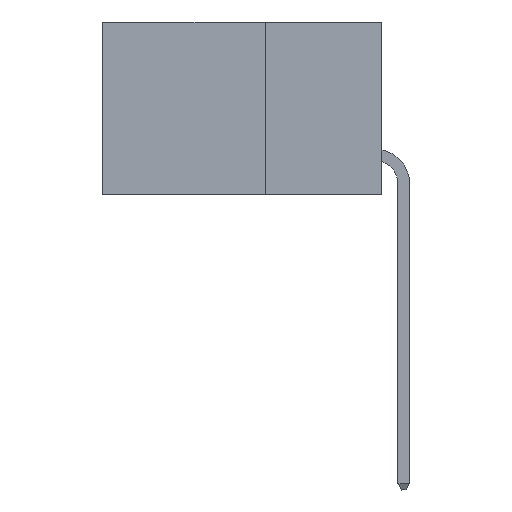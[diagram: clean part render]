
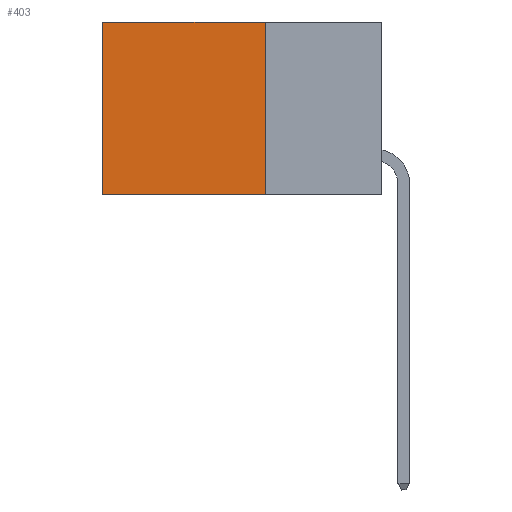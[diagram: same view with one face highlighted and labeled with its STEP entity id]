
A CAD part, left-side view. The second image highlights one B-rep face of the part: STEP entity #403.
In plain terms, the highlighted planar face has unit normal (-1, 0, 0).
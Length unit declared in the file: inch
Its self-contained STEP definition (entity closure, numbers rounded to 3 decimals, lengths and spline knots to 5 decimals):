
#159 = VERTEX_POINT ( 'NONE', #13754 ) ;
#403 = ADVANCED_FACE ( 'NONE', ( #7611 ), #3947, .F. ) ;
#595 = DIRECTION ( 'NONE',  ( 0., 0., -1. ) ) ;
#725 = DIRECTION ( 'NONE',  ( 1., 0., 0. ) ) ;
#1408 = VERTEX_POINT ( 'NONE', #18334 ) ;
#2193 = DIRECTION ( 'NONE',  ( 0., 0., -1. ) ) ;
#3204 = AXIS2_PLACEMENT_3D ( 'NONE', #6863, #725, #595 ) ;
#3571 = VECTOR ( 'NONE', #10130, 39.37008 ) ;
#3947 = PLANE ( 'NONE',  #3204 ) ;
#4691 = ORIENTED_EDGE ( 'NONE', *, *, #5246, .T. ) ;
#4752 = ORIENTED_EDGE ( 'NONE', *, *, #5936, .F. ) ;
#5246 = EDGE_CURVE ( 'NONE', #159, #1408, #19019, .T. ) ;
#5570 = LINE ( 'NONE', #14138, #19491 ) ;
#5896 = EDGE_LOOP ( 'NONE', ( #15686, #10786, #4752, #4691 ) ) ;
#5936 = EDGE_CURVE ( 'NONE', #159, #8295, #5570, .T. ) ;
#6798 = EDGE_CURVE ( 'NONE', #8295, #16236, #13762, .T. ) ;
#6863 = CARTESIAN_POINT ( 'NONE',  ( 0.2875, 0.25, 0. ) ) ;
#6903 = VECTOR ( 'NONE', #2193, 39.37008 ) ;
#7611 = FACE_OUTER_BOUND ( 'NONE', #5896, .T. ) ;
#8295 = VERTEX_POINT ( 'NONE', #10831 ) ;
#9796 = EDGE_CURVE ( 'NONE', #1408, #16236, #14875, .T. ) ;
#10130 = DIRECTION ( 'NONE',  ( 0., 1., 0. ) ) ;
#10323 = CARTESIAN_POINT ( 'NONE',  ( 0.2875, 0.25, -0.37 ) ) ;
#10786 = ORIENTED_EDGE ( 'NONE', *, *, #6798, .F. ) ;
#10831 = CARTESIAN_POINT ( 'NONE',  ( 0.2875, 0.25, -0.37 ) ) ;
#13754 = CARTESIAN_POINT ( 'NONE',  ( 0.2875, 0.25, 0. ) ) ;
#13762 = LINE ( 'NONE', #10323, #3571 ) ;
#14138 = CARTESIAN_POINT ( 'NONE',  ( 0.2875, 0.25, 0. ) ) ;
#14875 = LINE ( 'NONE', #16547, #6903 ) ;
#15065 = VECTOR ( 'NONE', #20376, 39.37008 ) ;
#15271 = CARTESIAN_POINT ( 'NONE',  ( 0.2875, 0.25, 0. ) ) ;
#15510 = DIRECTION ( 'NONE',  ( 0., 0., -1. ) ) ;
#15654 = CARTESIAN_POINT ( 'NONE',  ( 0.2875, 0.6, -0.37 ) ) ;
#15686 = ORIENTED_EDGE ( 'NONE', *, *, #9796, .T. ) ;
#16236 = VERTEX_POINT ( 'NONE', #15654 ) ;
#16547 = CARTESIAN_POINT ( 'NONE',  ( 0.2875, 0.6, 0. ) ) ;
#18334 = CARTESIAN_POINT ( 'NONE',  ( 0.2875, 0.6, 0. ) ) ;
#19019 = LINE ( 'NONE', #15271, #15065 ) ;
#19491 = VECTOR ( 'NONE', #15510, 39.37008 ) ;
#20376 = DIRECTION ( 'NONE',  ( 0., 1., 0. ) ) ;
